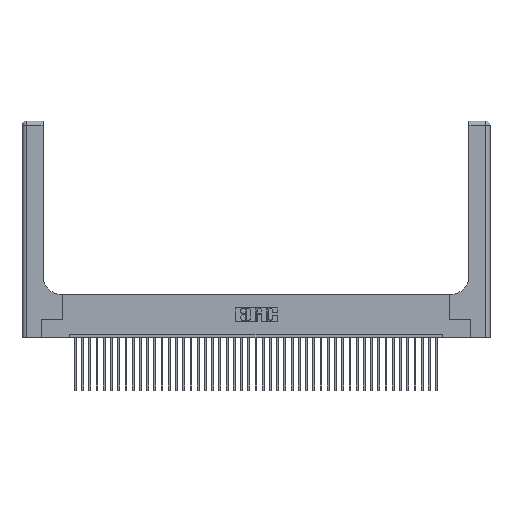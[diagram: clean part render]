
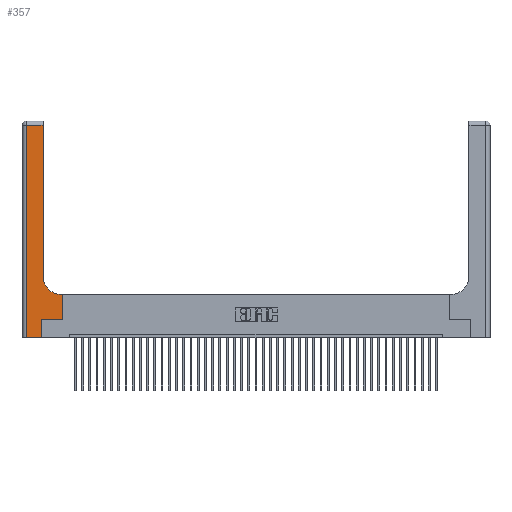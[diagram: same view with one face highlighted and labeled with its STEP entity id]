
A CAD part, top view. The second image highlights one B-rep face of the part: STEP entity #357.
In plain terms, the highlighted planar face has unit normal (0, 0, 1).
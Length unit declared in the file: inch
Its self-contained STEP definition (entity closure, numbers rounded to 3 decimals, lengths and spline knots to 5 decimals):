
#357 = ADVANCED_FACE ( 'NONE', ( #41592 ), #9113, .F. ) ;
#1941 = CARTESIAN_POINT ( 'NONE',  ( 0.06, 0., 0.37 ) ) ;
#3698 = DIRECTION ( 'NONE',  ( 0., 1., 0. ) ) ;
#3753 = VERTEX_POINT ( 'NONE', #25267 ) ;
#5081 = VECTOR ( 'NONE', #31731, 39.37008 ) ;
#6093 = VECTOR ( 'NONE', #30995, 39.37008 ) ;
#6568 = VERTEX_POINT ( 'NONE', #23226 ) ;
#7172 = EDGE_LOOP ( 'NONE', ( #30316, #12290, #40980, #13203, #42026, #9342, #37224, #22420, #26471 ) ) ;
#7570 = DIRECTION ( 'NONE',  ( 1., 0., 0. ) ) ;
#8015 = VERTEX_POINT ( 'NONE', #11296 ) ;
#9113 = PLANE ( 'NONE',  #15841 ) ;
#9248 = VERTEX_POINT ( 'NONE', #41241 ) ;
#9342 = ORIENTED_EDGE ( 'NONE', *, *, #32203, .T. ) ;
#9568 = VERTEX_POINT ( 'NONE', #9977 ) ;
#9832 = VERTEX_POINT ( 'NONE', #34365 ) ;
#9977 = CARTESIAN_POINT ( 'NONE',  ( 0.2915, 0.85, 0.37 ) ) ;
#10323 = AXIS2_PLACEMENT_3D ( 'NONE', #31435, #34876, #31146 ) ;
#10628 = LINE ( 'NONE', #26264, #22490 ) ;
#10821 = EDGE_CURVE ( 'NONE', #9248, #21465, #33659, .T. ) ;
#10922 = EDGE_CURVE ( 'NONE', #6568, #9568, #22498, .T. ) ;
#10964 = EDGE_CURVE ( 'NONE', #13226, #3753, #13718, .T. ) ;
#11296 = CARTESIAN_POINT ( 'NONE',  ( 0.2915, 2.94, 0.37 ) ) ;
#12057 = VECTOR ( 'NONE', #3698, 39.37008 ) ;
#12290 = ORIENTED_EDGE ( 'NONE', *, *, #27495, .T. ) ;
#13203 = ORIENTED_EDGE ( 'NONE', *, *, #23616, .T. ) ;
#13226 = VERTEX_POINT ( 'NONE', #24192 ) ;
#13718 = LINE ( 'NONE', #35029, #5081 ) ;
#15841 = AXIS2_PLACEMENT_3D ( 'NONE', #35456, #19007, #38623 ) ;
#16191 = LINE ( 'NONE', #26729, #12057 ) ;
#16339 = CARTESIAN_POINT ( 'NONE',  ( 0., 0., 0.37 ) ) ;
#16349 = VECTOR ( 'NONE', #31193, 39.37008 ) ;
#16491 = EDGE_CURVE ( 'NONE', #28954, #9832, #25072, .T. ) ;
#18110 = CARTESIAN_POINT ( 'NONE',  ( 0.269, 0., 0.37 ) ) ;
#19007 = DIRECTION ( 'NONE',  ( 0., 0., -1. ) ) ;
#21465 = VERTEX_POINT ( 'NONE', #1941 ) ;
#22314 = VECTOR ( 'NONE', #39258, 39.37008 ) ;
#22420 = ORIENTED_EDGE ( 'NONE', *, *, #23194, .T. ) ;
#22490 = VECTOR ( 'NONE', #25974, 39.37008 ) ;
#22498 = CIRCLE ( 'NONE', #10323, 0.25 ) ;
#23194 = EDGE_CURVE ( 'NONE', #3753, #6568, #40729, .T. ) ;
#23226 = CARTESIAN_POINT ( 'NONE',  ( 0.5415, 0.6, 0.37 ) ) ;
#23471 = VECTOR ( 'NONE', #7570, 39.37008 ) ;
#23616 = EDGE_CURVE ( 'NONE', #21465, #28954, #38150, .T. ) ;
#24192 = CARTESIAN_POINT ( 'NONE',  ( 0.5585, 0.25, 0.37 ) ) ;
#25072 = LINE ( 'NONE', #27758, #16349 ) ;
#25267 = CARTESIAN_POINT ( 'NONE',  ( 0.5585, 0.6, 0.37 ) ) ;
#25974 = DIRECTION ( 'NONE',  ( -1., 0., 0. ) ) ;
#26125 = CARTESIAN_POINT ( 'NONE',  ( 0.2915, 0.6, 0.37 ) ) ;
#26264 = CARTESIAN_POINT ( 'NONE',  ( 0., 2.94, 0.37 ) ) ;
#26471 = ORIENTED_EDGE ( 'NONE', *, *, #10922, .T. ) ;
#26729 = CARTESIAN_POINT ( 'NONE',  ( 0.2915, 3., 0.37 ) ) ;
#27189 = CARTESIAN_POINT ( 'NONE',  ( 0.269, 0.25, 0.37 ) ) ;
#27495 = EDGE_CURVE ( 'NONE', #8015, #9248, #10628, .T. ) ;
#27758 = CARTESIAN_POINT ( 'NONE',  ( 0.269, 0., 0.37 ) ) ;
#28954 = VERTEX_POINT ( 'NONE', #18110 ) ;
#29412 = VECTOR ( 'NONE', #38955, 39.37008 ) ;
#30316 = ORIENTED_EDGE ( 'NONE', *, *, #40709, .T. ) ;
#30995 = DIRECTION ( 'NONE',  ( 0., -1., 0. ) ) ;
#31146 = DIRECTION ( 'NONE',  ( 1., 0., 0. ) ) ;
#31193 = DIRECTION ( 'NONE',  ( 0., 1., 0. ) ) ;
#31435 = CARTESIAN_POINT ( 'NONE',  ( 0.5415, 0.85, 0.37 ) ) ;
#31731 = DIRECTION ( 'NONE',  ( 0., 1., 0. ) ) ;
#32203 = EDGE_CURVE ( 'NONE', #9832, #13226, #32664, .T. ) ;
#32664 = LINE ( 'NONE', #27189, #23471 ) ;
#33659 = LINE ( 'NONE', #34005, #6093 ) ;
#34005 = CARTESIAN_POINT ( 'NONE',  ( 0.06, 3., 0.37 ) ) ;
#34365 = CARTESIAN_POINT ( 'NONE',  ( 0.269, 0.25, 0.37 ) ) ;
#34876 = DIRECTION ( 'NONE',  ( 0., 0., -1. ) ) ;
#35029 = CARTESIAN_POINT ( 'NONE',  ( 0.5585, 0.25, 0.37 ) ) ;
#35456 = CARTESIAN_POINT ( 'NONE',  ( 0., 3., 0.37 ) ) ;
#37224 = ORIENTED_EDGE ( 'NONE', *, *, #10964, .T. ) ;
#38150 = LINE ( 'NONE', #16339, #29412 ) ;
#38623 = DIRECTION ( 'NONE',  ( -1., 0., 0. ) ) ;
#38955 = DIRECTION ( 'NONE',  ( 1., 0., 0. ) ) ;
#39258 = DIRECTION ( 'NONE',  ( -1., 0., 0. ) ) ;
#40709 = EDGE_CURVE ( 'NONE', #9568, #8015, #16191, .T. ) ;
#40729 = LINE ( 'NONE', #26125, #22314 ) ;
#40980 = ORIENTED_EDGE ( 'NONE', *, *, #10821, .T. ) ;
#41241 = CARTESIAN_POINT ( 'NONE',  ( 0.06, 2.94, 0.37 ) ) ;
#41592 = FACE_OUTER_BOUND ( 'NONE', #7172, .T. ) ;
#42026 = ORIENTED_EDGE ( 'NONE', *, *, #16491, .T. ) ;
